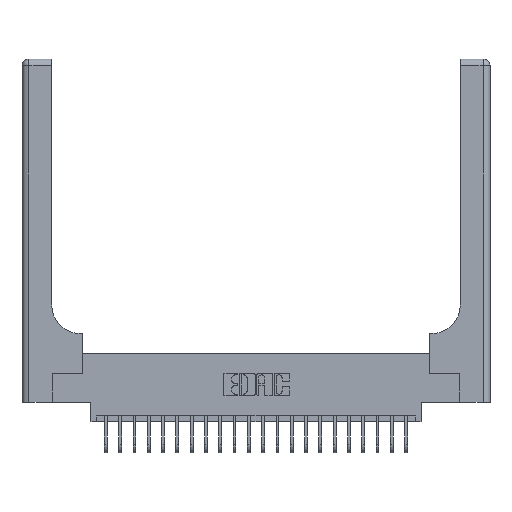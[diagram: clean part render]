
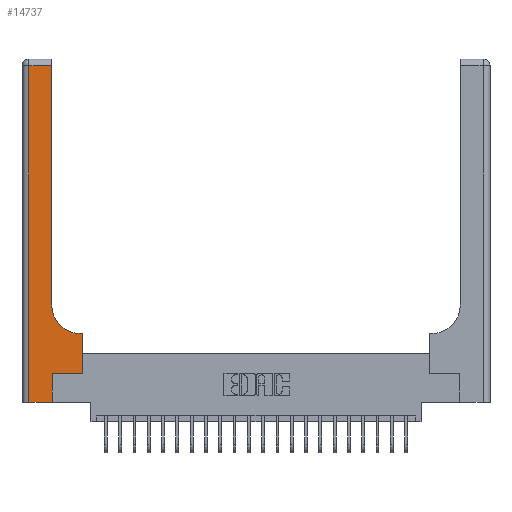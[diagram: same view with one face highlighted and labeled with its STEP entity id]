
A CAD part, top view. The second image highlights one B-rep face of the part: STEP entity #14737.
In plain terms, the highlighted planar face has unit normal (0, 0, 1).
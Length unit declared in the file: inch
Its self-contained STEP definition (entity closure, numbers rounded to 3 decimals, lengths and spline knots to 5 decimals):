
#716 = DIRECTION ( 'NONE',  ( 0., 0., -1. ) ) ;
#975 = EDGE_CURVE ( 'NONE', #3349, #15841, #1811, .T. ) ;
#1596 = PLANE ( 'NONE',  #9298 ) ;
#1605 = ORIENTED_EDGE ( 'NONE', *, *, #975, .T. ) ;
#1811 = LINE ( 'NONE', #15345, #15985 ) ;
#1837 = ORIENTED_EDGE ( 'NONE', *, *, #14211, .T. ) ;
#2057 = VECTOR ( 'NONE', #20031, 39.37008 ) ;
#2450 = EDGE_CURVE ( 'NONE', #14647, #3349, #5393, .T. ) ;
#2749 = LINE ( 'NONE', #4731, #2057 ) ;
#2790 = LINE ( 'NONE', #19462, #4377 ) ;
#2980 = ORIENTED_EDGE ( 'NONE', *, *, #21700, .T. ) ;
#3084 = CARTESIAN_POINT ( 'NONE',  ( 0.06, 2.94, 0.37 ) ) ;
#3274 = CARTESIAN_POINT ( 'NONE',  ( 0., 2.94, 0.37 ) ) ;
#3349 = VERTEX_POINT ( 'NONE', #3084 ) ;
#3661 = EDGE_CURVE ( 'NONE', #4162, #20012, #15624, .T. ) ;
#4162 = VERTEX_POINT ( 'NONE', #19705 ) ;
#4377 = VECTOR ( 'NONE', #17952, 39.37008 ) ;
#4731 = CARTESIAN_POINT ( 'NONE',  ( 0.26, 3., 0.37 ) ) ;
#5114 = DIRECTION ( 'NONE',  ( 0., 1., 0. ) ) ;
#5393 = LINE ( 'NONE', #3274, #19638 ) ;
#5458 = DIRECTION ( 'NONE',  ( -1., 0., 0. ) ) ;
#5570 = EDGE_LOOP ( 'NONE', ( #8152, #16947, #1605, #14043, #6703, #7610, #1837, #22604, #2980 ) ) ;
#5586 = DIRECTION ( 'NONE',  ( 0., 0., -1. ) ) ;
#5674 = DIRECTION ( 'NONE',  ( 0., -1., 0. ) ) ;
#5766 = CARTESIAN_POINT ( 'NONE',  ( 0.528, 0.25, 0.37 ) ) ;
#6491 = CARTESIAN_POINT ( 'NONE',  ( 0.06, 0., 0.37 ) ) ;
#6703 = ORIENTED_EDGE ( 'NONE', *, *, #3661, .T. ) ;
#6982 = CARTESIAN_POINT ( 'NONE',  ( 0.528, 0.25, 0.37 ) ) ;
#7610 = ORIENTED_EDGE ( 'NONE', *, *, #22484, .T. ) ;
#7832 = VECTOR ( 'NONE', #7924, 39.37008 ) ;
#7924 = DIRECTION ( 'NONE',  ( 0., 1., 0. ) ) ;
#8152 = ORIENTED_EDGE ( 'NONE', *, *, #10255, .T. ) ;
#9282 = VECTOR ( 'NONE', #5114, 39.37008 ) ;
#9298 = AXIS2_PLACEMENT_3D ( 'NONE', #15018, #5586, #5458 ) ;
#10079 = EDGE_CURVE ( 'NONE', #15841, #4162, #17415, .T. ) ;
#10255 = EDGE_CURVE ( 'NONE', #19088, #14647, #2749, .T. ) ;
#10893 = EDGE_CURVE ( 'NONE', #21289, #22621, #23687, .T. ) ;
#11588 = CARTESIAN_POINT ( 'NONE',  ( 0., 0., 0.37 ) ) ;
#11657 = CARTESIAN_POINT ( 'NONE',  ( 0.265, 0., 0.37 ) ) ;
#13460 = CARTESIAN_POINT ( 'NONE',  ( 0.528, 0.6, 0.37 ) ) ;
#13586 = VECTOR ( 'NONE', #19820, 39.37008 ) ;
#13635 = CARTESIAN_POINT ( 'NONE',  ( 0.26, 0.85, 0.37 ) ) ;
#14043 = ORIENTED_EDGE ( 'NONE', *, *, #10079, .T. ) ;
#14211 = EDGE_CURVE ( 'NONE', #19964, #21289, #22156, .T. ) ;
#14647 = VERTEX_POINT ( 'NONE', #20013 ) ;
#14737 = ADVANCED_FACE ( 'NONE', ( #20423 ), #1596, .F. ) ;
#14741 = VECTOR ( 'NONE', #23283, 39.37008 ) ;
#15018 = CARTESIAN_POINT ( 'NONE',  ( 0., 3., 0.37 ) ) ;
#15345 = CARTESIAN_POINT ( 'NONE',  ( 0.06, 3., 0.37 ) ) ;
#15624 = LINE ( 'NONE', #11657, #7832 ) ;
#15841 = VERTEX_POINT ( 'NONE', #6491 ) ;
#15985 = VECTOR ( 'NONE', #5674, 39.37008 ) ;
#16947 = ORIENTED_EDGE ( 'NONE', *, *, #2450, .T. ) ;
#17415 = LINE ( 'NONE', #11588, #14741 ) ;
#17755 = DIRECTION ( 'NONE',  ( 1., 0., 0. ) ) ;
#17952 = DIRECTION ( 'NONE',  ( 1., 0., 0. ) ) ;
#19088 = VERTEX_POINT ( 'NONE', #13635 ) ;
#19285 = CARTESIAN_POINT ( 'NONE',  ( 0.51, 0.85, 0.37 ) ) ;
#19462 = CARTESIAN_POINT ( 'NONE',  ( 0.265, 0.25, 0.37 ) ) ;
#19638 = VECTOR ( 'NONE', #20553, 39.37008 ) ;
#19705 = CARTESIAN_POINT ( 'NONE',  ( 0.265, 0., 0.37 ) ) ;
#19820 = DIRECTION ( 'NONE',  ( -1., 0., 0. ) ) ;
#19851 = CIRCLE ( 'NONE', #20249, 0.25 ) ;
#19947 = CARTESIAN_POINT ( 'NONE',  ( 0.51, 0.6, 0.37 ) ) ;
#19964 = VERTEX_POINT ( 'NONE', #5766 ) ;
#20012 = VERTEX_POINT ( 'NONE', #22674 ) ;
#20013 = CARTESIAN_POINT ( 'NONE',  ( 0.26, 2.94, 0.37 ) ) ;
#20031 = DIRECTION ( 'NONE',  ( 0., 1., 0. ) ) ;
#20249 = AXIS2_PLACEMENT_3D ( 'NONE', #19285, #716, #17755 ) ;
#20423 = FACE_OUTER_BOUND ( 'NONE', #5570, .T. ) ;
#20553 = DIRECTION ( 'NONE',  ( -1., 0., 0. ) ) ;
#21289 = VERTEX_POINT ( 'NONE', #13460 ) ;
#21324 = CARTESIAN_POINT ( 'NONE',  ( 0.26, 0.6, 0.37 ) ) ;
#21700 = EDGE_CURVE ( 'NONE', #22621, #19088, #19851, .T. ) ;
#22156 = LINE ( 'NONE', #6982, #9282 ) ;
#22484 = EDGE_CURVE ( 'NONE', #20012, #19964, #2790, .T. ) ;
#22604 = ORIENTED_EDGE ( 'NONE', *, *, #10893, .T. ) ;
#22621 = VERTEX_POINT ( 'NONE', #19947 ) ;
#22674 = CARTESIAN_POINT ( 'NONE',  ( 0.265, 0.25, 0.37 ) ) ;
#23283 = DIRECTION ( 'NONE',  ( 1., 0., 0. ) ) ;
#23687 = LINE ( 'NONE', #21324, #13586 ) ;
